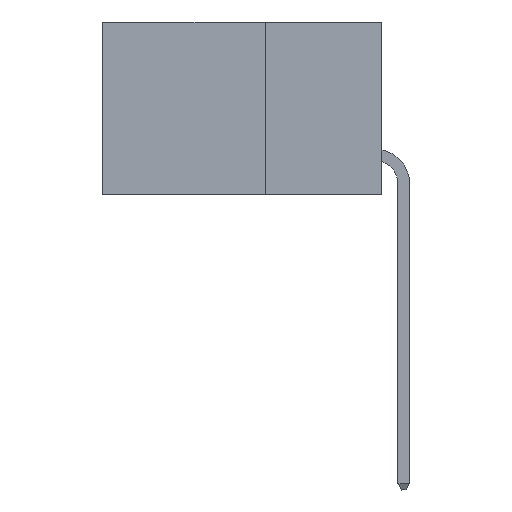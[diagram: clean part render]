
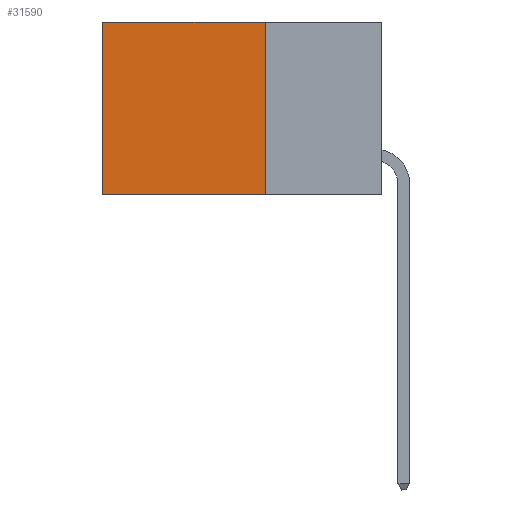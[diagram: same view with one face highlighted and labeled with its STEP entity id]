
A CAD part, left-side view. The second image highlights one B-rep face of the part: STEP entity #31590.
In plain terms, the highlighted planar face has unit normal (-1, 0, 0).
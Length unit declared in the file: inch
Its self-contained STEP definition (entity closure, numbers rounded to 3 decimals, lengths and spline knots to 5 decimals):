
#2768 = LINE ( 'NONE', #34380, #33878 ) ;
#3390 = EDGE_CURVE ( 'NONE', #35320, #19821, #37959, .T. ) ;
#3567 = CARTESIAN_POINT ( 'NONE',  ( 0.2875, 0.25, 0. ) ) ;
#4407 = LINE ( 'NONE', #40265, #43202 ) ;
#5928 = CARTESIAN_POINT ( 'NONE',  ( 0.2875, 0.25, -0.37 ) ) ;
#7026 = VERTEX_POINT ( 'NONE', #5928 ) ;
#8594 = EDGE_CURVE ( 'NONE', #19821, #37077, #4407, .T. ) ;
#10403 = ORIENTED_EDGE ( 'NONE', *, *, #37266, .F. ) ;
#11207 = DIRECTION ( 'NONE',  ( 0., 1., 0. ) ) ;
#11595 = ORIENTED_EDGE ( 'NONE', *, *, #3390, .T. ) ;
#18632 = AXIS2_PLACEMENT_3D ( 'NONE', #43476, #42793, #42955 ) ;
#19821 = VERTEX_POINT ( 'NONE', #24051 ) ;
#21761 = VECTOR ( 'NONE', #31127, 39.37008 ) ;
#23145 = ORIENTED_EDGE ( 'NONE', *, *, #37088, .F. ) ;
#24051 = CARTESIAN_POINT ( 'NONE',  ( 0.2875, 0.6, 0. ) ) ;
#25170 = DIRECTION ( 'NONE',  ( 0., 0., -1. ) ) ;
#26714 = EDGE_LOOP ( 'NONE', ( #39160, #10403, #23145, #11595 ) ) ;
#27398 = FACE_OUTER_BOUND ( 'NONE', #26714, .T. ) ;
#28278 = CARTESIAN_POINT ( 'NONE',  ( 0.2875, 0.6, -0.37 ) ) ;
#30393 = CARTESIAN_POINT ( 'NONE',  ( 0.2875, 0.25, -0.37 ) ) ;
#30763 = LINE ( 'NONE', #30393, #41610 ) ;
#31127 = DIRECTION ( 'NONE',  ( 0., 1., 0. ) ) ;
#31590 = ADVANCED_FACE ( 'NONE', ( #27398 ), #35808, .F. ) ;
#33878 = VECTOR ( 'NONE', #43392, 39.37008 ) ;
#34380 = CARTESIAN_POINT ( 'NONE',  ( 0.2875, 0.25, 0. ) ) ;
#35320 = VERTEX_POINT ( 'NONE', #3567 ) ;
#35808 = PLANE ( 'NONE',  #18632 ) ;
#36476 = CARTESIAN_POINT ( 'NONE',  ( 0.2875, 0.25, 0. ) ) ;
#37077 = VERTEX_POINT ( 'NONE', #28278 ) ;
#37088 = EDGE_CURVE ( 'NONE', #35320, #7026, #2768, .T. ) ;
#37266 = EDGE_CURVE ( 'NONE', #7026, #37077, #30763, .T. ) ;
#37959 = LINE ( 'NONE', #36476, #21761 ) ;
#39160 = ORIENTED_EDGE ( 'NONE', *, *, #8594, .T. ) ;
#40265 = CARTESIAN_POINT ( 'NONE',  ( 0.2875, 0.6, 0. ) ) ;
#41610 = VECTOR ( 'NONE', #11207, 39.37008 ) ;
#42793 = DIRECTION ( 'NONE',  ( 1., 0., 0. ) ) ;
#42955 = DIRECTION ( 'NONE',  ( 0., 0., -1. ) ) ;
#43202 = VECTOR ( 'NONE', #25170, 39.37008 ) ;
#43392 = DIRECTION ( 'NONE',  ( 0., 0., -1. ) ) ;
#43476 = CARTESIAN_POINT ( 'NONE',  ( 0.2875, 0.25, 0. ) ) ;
